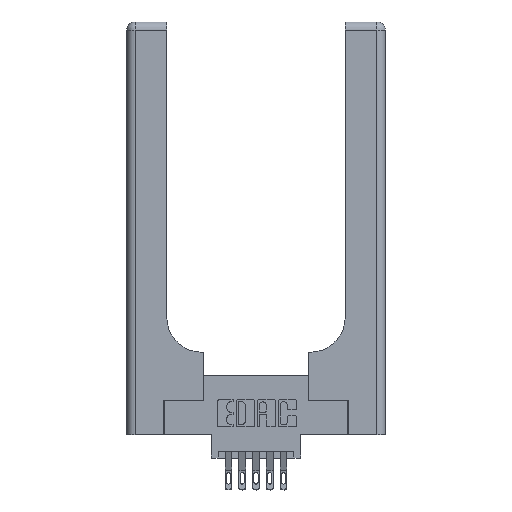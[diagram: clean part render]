
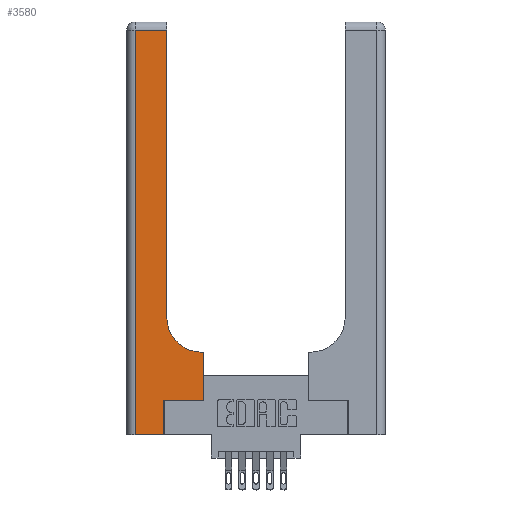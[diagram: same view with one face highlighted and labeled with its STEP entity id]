
A CAD part, top view. The second image highlights one B-rep face of the part: STEP entity #3580.
In plain terms, the highlighted planar face has unit normal (0, 0, 1).
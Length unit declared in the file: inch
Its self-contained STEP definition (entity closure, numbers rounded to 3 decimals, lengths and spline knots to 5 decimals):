
#13 = DIRECTION ( 'NONE',  ( 1., 0., 0. ) ) ;
#155 = CARTESIAN_POINT ( 'NONE',  ( 0.5415, 0.6, 0.37 ) ) ;
#417 = EDGE_CURVE ( 'NONE', #7244, #3218, #1486, .T. ) ;
#471 = EDGE_CURVE ( 'NONE', #10255, #7576, #7296, .T. ) ;
#487 = DIRECTION ( 'NONE',  ( 1., 0., 0. ) ) ;
#653 = CARTESIAN_POINT ( 'NONE',  ( 0.5585, 0.25, 0.37 ) ) ;
#780 = VECTOR ( 'NONE', #13, 39.37008 ) ;
#791 = CARTESIAN_POINT ( 'NONE',  ( 0.06, 2.94, 0.37 ) ) ;
#834 = CARTESIAN_POINT ( 'NONE',  ( 0.2915, 0.85, 0.37 ) ) ;
#1095 = EDGE_LOOP ( 'NONE', ( #1218, #5014, #3213, #9508, #11885, #5560, #5372, #6300, #10689 ) ) ;
#1218 = ORIENTED_EDGE ( 'NONE', *, *, #7148, .T. ) ;
#1293 = CARTESIAN_POINT ( 'NONE',  ( 0.5415, 0.85, 0.37 ) ) ;
#1307 = VECTOR ( 'NONE', #4622, 39.37008 ) ;
#1486 = LINE ( 'NONE', #2358, #1307 ) ;
#1605 = LINE ( 'NONE', #11863, #8306 ) ;
#1716 = LINE ( 'NONE', #4657, #10512 ) ;
#2306 = DIRECTION ( 'NONE',  ( -1., 0., 0. ) ) ;
#2314 = VERTEX_POINT ( 'NONE', #155 ) ;
#2358 = CARTESIAN_POINT ( 'NONE',  ( 0.269, 0., 0.37 ) ) ;
#3015 = EDGE_CURVE ( 'NONE', #13009, #7244, #7562, .T. ) ;
#3213 = ORIENTED_EDGE ( 'NONE', *, *, #4011, .T. ) ;
#3218 = VERTEX_POINT ( 'NONE', #9019 ) ;
#3283 = PLANE ( 'NONE',  #11596 ) ;
#3537 = VECTOR ( 'NONE', #2306, 39.37008 ) ;
#3580 = ADVANCED_FACE ( 'NONE', ( #12567 ), #3283, .F. ) ;
#3739 = EDGE_CURVE ( 'NONE', #2314, #8337, #10274, .T. ) ;
#4011 = EDGE_CURVE ( 'NONE', #12138, #13009, #5322, .T. ) ;
#4570 = CARTESIAN_POINT ( 'NONE',  ( 0., 2.94, 0.37 ) ) ;
#4622 = DIRECTION ( 'NONE',  ( 0., 1., 0. ) ) ;
#4657 = CARTESIAN_POINT ( 'NONE',  ( 0.2915, 3., 0.37 ) ) ;
#5011 = AXIS2_PLACEMENT_3D ( 'NONE', #1293, #9178, #11745 ) ;
#5014 = ORIENTED_EDGE ( 'NONE', *, *, #6533, .T. ) ;
#5188 = LINE ( 'NONE', #12458, #780 ) ;
#5322 = LINE ( 'NONE', #7397, #6398 ) ;
#5372 = ORIENTED_EDGE ( 'NONE', *, *, #471, .T. ) ;
#5510 = DIRECTION ( 'NONE',  ( 0., 0., -1. ) ) ;
#5513 = CARTESIAN_POINT ( 'NONE',  ( 0.5585, 0.6, 0.37 ) ) ;
#5560 = ORIENTED_EDGE ( 'NONE', *, *, #11886, .T. ) ;
#5578 = VERTEX_POINT ( 'NONE', #13547 ) ;
#6300 = ORIENTED_EDGE ( 'NONE', *, *, #13844, .T. ) ;
#6398 = VECTOR ( 'NONE', #11855, 39.37008 ) ;
#6533 = EDGE_CURVE ( 'NONE', #5578, #12138, #9488, .T. ) ;
#6849 = CARTESIAN_POINT ( 'NONE',  ( 0.5585, 0.25, 0.37 ) ) ;
#7148 = EDGE_CURVE ( 'NONE', #8337, #5578, #1716, .T. ) ;
#7244 = VERTEX_POINT ( 'NONE', #8287 ) ;
#7296 = LINE ( 'NONE', #653, #12573 ) ;
#7397 = CARTESIAN_POINT ( 'NONE',  ( 0.06, 3., 0.37 ) ) ;
#7562 = LINE ( 'NONE', #12788, #10015 ) ;
#7576 = VERTEX_POINT ( 'NONE', #5513 ) ;
#7994 = DIRECTION ( 'NONE',  ( 0., 1., 0. ) ) ;
#8287 = CARTESIAN_POINT ( 'NONE',  ( 0.269, 0., 0.37 ) ) ;
#8306 = VECTOR ( 'NONE', #13040, 39.37008 ) ;
#8337 = VERTEX_POINT ( 'NONE', #834 ) ;
#9019 = CARTESIAN_POINT ( 'NONE',  ( 0.269, 0.25, 0.37 ) ) ;
#9110 = CARTESIAN_POINT ( 'NONE',  ( 0.06, 0., 0.37 ) ) ;
#9178 = DIRECTION ( 'NONE',  ( 0., 0., -1. ) ) ;
#9488 = LINE ( 'NONE', #4570, #3537 ) ;
#9508 = ORIENTED_EDGE ( 'NONE', *, *, #3015, .T. ) ;
#10015 = VECTOR ( 'NONE', #487, 39.37008 ) ;
#10255 = VERTEX_POINT ( 'NONE', #6849 ) ;
#10274 = CIRCLE ( 'NONE', #5011, 0.25 ) ;
#10512 = VECTOR ( 'NONE', #7994, 39.37008 ) ;
#10689 = ORIENTED_EDGE ( 'NONE', *, *, #3739, .T. ) ;
#10838 = DIRECTION ( 'NONE',  ( 0., 1., 0. ) ) ;
#11596 = AXIS2_PLACEMENT_3D ( 'NONE', #13531, #5510, #14493 ) ;
#11745 = DIRECTION ( 'NONE',  ( 1., 0., 0. ) ) ;
#11855 = DIRECTION ( 'NONE',  ( 0., -1., 0. ) ) ;
#11863 = CARTESIAN_POINT ( 'NONE',  ( 0.2915, 0.6, 0.37 ) ) ;
#11885 = ORIENTED_EDGE ( 'NONE', *, *, #417, .T. ) ;
#11886 = EDGE_CURVE ( 'NONE', #3218, #10255, #5188, .T. ) ;
#12138 = VERTEX_POINT ( 'NONE', #791 ) ;
#12458 = CARTESIAN_POINT ( 'NONE',  ( 0.269, 0.25, 0.37 ) ) ;
#12567 = FACE_OUTER_BOUND ( 'NONE', #1095, .T. ) ;
#12573 = VECTOR ( 'NONE', #10838, 39.37008 ) ;
#12788 = CARTESIAN_POINT ( 'NONE',  ( 0., 0., 0.37 ) ) ;
#13009 = VERTEX_POINT ( 'NONE', #9110 ) ;
#13040 = DIRECTION ( 'NONE',  ( -1., 0., 0. ) ) ;
#13531 = CARTESIAN_POINT ( 'NONE',  ( 0., 3., 0.37 ) ) ;
#13547 = CARTESIAN_POINT ( 'NONE',  ( 0.2915, 2.94, 0.37 ) ) ;
#13844 = EDGE_CURVE ( 'NONE', #7576, #2314, #1605, .T. ) ;
#14493 = DIRECTION ( 'NONE',  ( -1., 0., 0. ) ) ;
